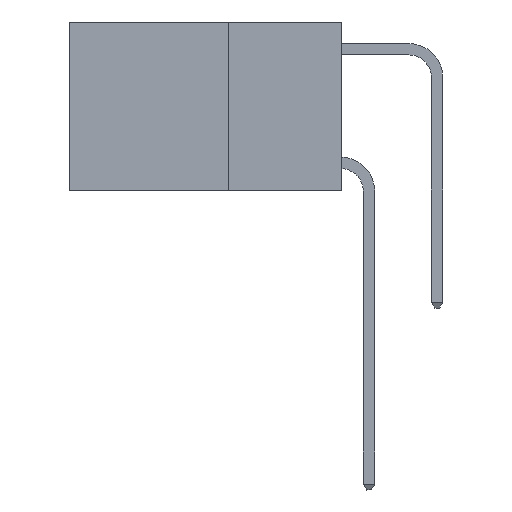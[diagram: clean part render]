
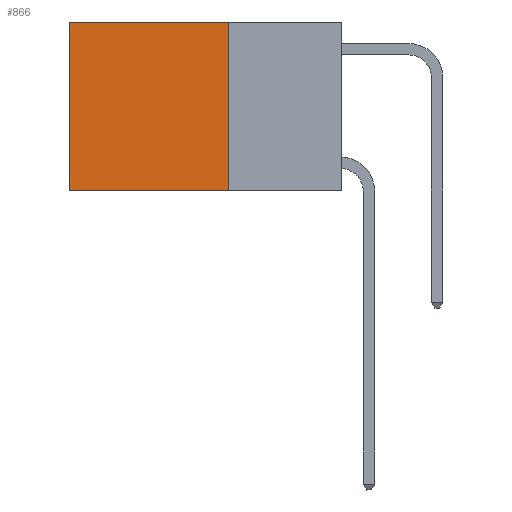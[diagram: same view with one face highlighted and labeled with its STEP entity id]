
A CAD part, left-side view. The second image highlights one B-rep face of the part: STEP entity #866.
In plain terms, the highlighted planar face has unit normal (-1, 0, 0).
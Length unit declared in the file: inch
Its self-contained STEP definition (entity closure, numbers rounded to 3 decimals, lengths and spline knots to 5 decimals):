
#771 = LINE ( 'NONE', #2067, #8175 ) ;
#866 = ADVANCED_FACE ( 'NONE', ( #9463 ), #4911, .F. ) ;
#1339 = AXIS2_PLACEMENT_3D ( 'NONE', #4991, #5910, #5748 ) ;
#1748 = VECTOR ( 'NONE', #2919, 39.37008 ) ;
#2067 = CARTESIAN_POINT ( 'NONE',  ( 0.2625, 0.6, 0. ) ) ;
#2207 = VERTEX_POINT ( 'NONE', #5621 ) ;
#2657 = EDGE_CURVE ( 'NONE', #7621, #2945, #771, .T. ) ;
#2919 = DIRECTION ( 'NONE',  ( 0., 1., 0. ) ) ;
#2945 = VERTEX_POINT ( 'NONE', #4320 ) ;
#3235 = CARTESIAN_POINT ( 'NONE',  ( 0.2625, 0.6, 0. ) ) ;
#3378 = LINE ( 'NONE', #4139, #8295 ) ;
#3397 = ORIENTED_EDGE ( 'NONE', *, *, #5808, .T. ) ;
#3481 = ORIENTED_EDGE ( 'NONE', *, *, #2657, .T. ) ;
#4139 = CARTESIAN_POINT ( 'NONE',  ( 0.2625, 0.25, -0.37 ) ) ;
#4320 = CARTESIAN_POINT ( 'NONE',  ( 0.2625, 0.6, -0.37 ) ) ;
#4911 = PLANE ( 'NONE',  #1339 ) ;
#4991 = CARTESIAN_POINT ( 'NONE',  ( 0.2625, 0.25, 0. ) ) ;
#5590 = CARTESIAN_POINT ( 'NONE',  ( 0.2625, 0.25, 0. ) ) ;
#5621 = CARTESIAN_POINT ( 'NONE',  ( 0.2625, 0.25, -0.37 ) ) ;
#5748 = DIRECTION ( 'NONE',  ( 0., 0., -1. ) ) ;
#5808 = EDGE_CURVE ( 'NONE', #7493, #7621, #11684, .T. ) ;
#5910 = DIRECTION ( 'NONE',  ( 1., 0., 0. ) ) ;
#6095 = ORIENTED_EDGE ( 'NONE', *, *, #8050, .F. ) ;
#6807 = ORIENTED_EDGE ( 'NONE', *, *, #8355, .F. ) ;
#7436 = DIRECTION ( 'NONE',  ( 0., 0., -1. ) ) ;
#7448 = EDGE_LOOP ( 'NONE', ( #3481, #6807, #6095, #3397 ) ) ;
#7493 = VERTEX_POINT ( 'NONE', #10566 ) ;
#7621 = VERTEX_POINT ( 'NONE', #3235 ) ;
#8050 = EDGE_CURVE ( 'NONE', #7493, #2207, #8752, .T. ) ;
#8175 = VECTOR ( 'NONE', #8546, 39.37008 ) ;
#8295 = VECTOR ( 'NONE', #9757, 39.37008 ) ;
#8355 = EDGE_CURVE ( 'NONE', #2207, #2945, #3378, .T. ) ;
#8546 = DIRECTION ( 'NONE',  ( 0., 0., -1. ) ) ;
#8752 = LINE ( 'NONE', #5590, #11584 ) ;
#9463 = FACE_OUTER_BOUND ( 'NONE', #7448, .T. ) ;
#9757 = DIRECTION ( 'NONE',  ( 0., 1., 0. ) ) ;
#10566 = CARTESIAN_POINT ( 'NONE',  ( 0.2625, 0.25, 0. ) ) ;
#11334 = CARTESIAN_POINT ( 'NONE',  ( 0.2625, 0.25, 0. ) ) ;
#11584 = VECTOR ( 'NONE', #7436, 39.37008 ) ;
#11684 = LINE ( 'NONE', #11334, #1748 ) ;
